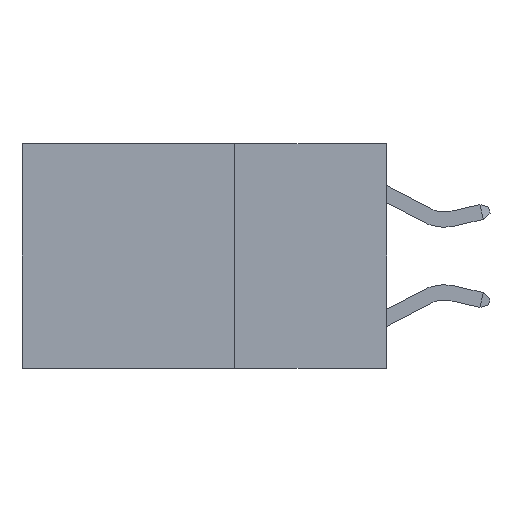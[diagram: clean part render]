
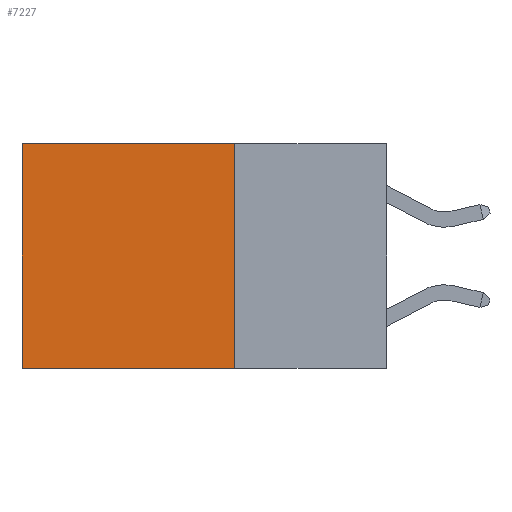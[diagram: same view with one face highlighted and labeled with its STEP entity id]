
A CAD part, left-side view. The second image highlights one B-rep face of the part: STEP entity #7227.
In plain terms, the highlighted planar face has unit normal (-1, 0, 0).
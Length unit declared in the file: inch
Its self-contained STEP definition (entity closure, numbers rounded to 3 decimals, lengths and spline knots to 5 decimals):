
#17 = FACE_OUTER_BOUND ( 'NONE', #5427, .T. ) ;
#21 = CARTESIAN_POINT ( 'NONE',  ( 0.2625, 0.25, 0. ) ) ;
#64 = EDGE_CURVE ( 'NONE', #10159, #2133, #747, .T. ) ;
#134 = VECTOR ( 'NONE', #7963, 39.37008 ) ;
#167 = EDGE_CURVE ( 'NONE', #2133, #10685, #7960, .T. ) ;
#476 = VERTEX_POINT ( 'NONE', #2195 ) ;
#747 = LINE ( 'NONE', #21, #6832 ) ;
#1163 = CARTESIAN_POINT ( 'NONE',  ( 0.2625, 0.6, -0.37 ) ) ;
#2049 = CARTESIAN_POINT ( 'NONE',  ( 0.2625, 0.6, 0. ) ) ;
#2133 = VERTEX_POINT ( 'NONE', #2049 ) ;
#2195 = CARTESIAN_POINT ( 'NONE',  ( 0.2625, 0.25, -0.37 ) ) ;
#2914 = EDGE_CURVE ( 'NONE', #10159, #476, #8668, .T. ) ;
#2926 = CARTESIAN_POINT ( 'NONE',  ( 0.2625, 0.25, 0. ) ) ;
#3120 = CARTESIAN_POINT ( 'NONE',  ( 0.2625, 0.25, 0. ) ) ;
#3753 = DIRECTION ( 'NONE',  ( 0., 0., -1. ) ) ;
#3911 = ORIENTED_EDGE ( 'NONE', *, *, #167, .T. ) ;
#4272 = ORIENTED_EDGE ( 'NONE', *, *, #2914, .F. ) ;
#5267 = CARTESIAN_POINT ( 'NONE',  ( 0.2625, 0.6, 0. ) ) ;
#5427 = EDGE_LOOP ( 'NONE', ( #3911, #6184, #4272, #8144 ) ) ;
#5809 = DIRECTION ( 'NONE',  ( 0., 1., 0. ) ) ;
#5811 = VECTOR ( 'NONE', #9262, 39.37008 ) ;
#6020 = DIRECTION ( 'NONE',  ( 0., 1., 0. ) ) ;
#6103 = VECTOR ( 'NONE', #6020, 39.37008 ) ;
#6184 = ORIENTED_EDGE ( 'NONE', *, *, #9061, .F. ) ;
#6832 = VECTOR ( 'NONE', #5809, 39.37008 ) ;
#7227 = ADVANCED_FACE ( 'NONE', ( #17 ), #9379, .F. ) ;
#7890 = CARTESIAN_POINT ( 'NONE',  ( 0.2625, 0.25, 0. ) ) ;
#7960 = LINE ( 'NONE', #5267, #5811 ) ;
#7963 = DIRECTION ( 'NONE',  ( 0., 0., -1. ) ) ;
#8144 = ORIENTED_EDGE ( 'NONE', *, *, #64, .T. ) ;
#8256 = LINE ( 'NONE', #9241, #6103 ) ;
#8604 = DIRECTION ( 'NONE',  ( 1., 0., 0. ) ) ;
#8668 = LINE ( 'NONE', #3120, #134 ) ;
#9061 = EDGE_CURVE ( 'NONE', #476, #10685, #8256, .T. ) ;
#9241 = CARTESIAN_POINT ( 'NONE',  ( 0.2625, 0.25, -0.37 ) ) ;
#9262 = DIRECTION ( 'NONE',  ( 0., 0., -1. ) ) ;
#9379 = PLANE ( 'NONE',  #9800 ) ;
#9800 = AXIS2_PLACEMENT_3D ( 'NONE', #2926, #8604, #3753 ) ;
#10159 = VERTEX_POINT ( 'NONE', #7890 ) ;
#10685 = VERTEX_POINT ( 'NONE', #1163 ) ;
